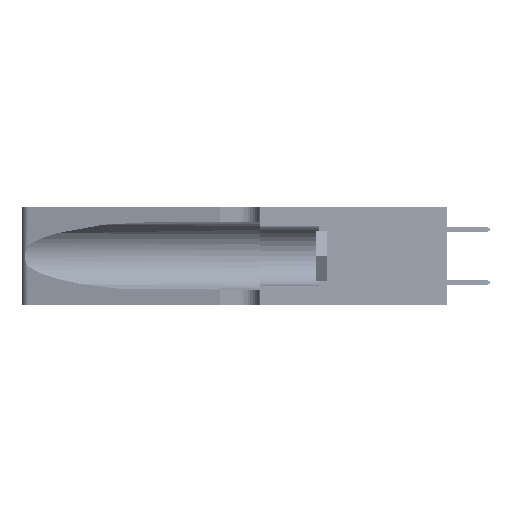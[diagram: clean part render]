
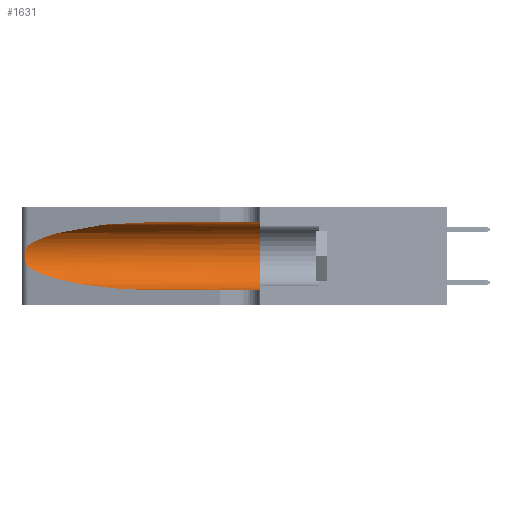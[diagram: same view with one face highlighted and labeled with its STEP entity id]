
A CAD part, left-side view. The second image highlights one B-rep face of the part: STEP entity #1631.
In plain terms, the highlighted cylindrical face has radius 3.308 mm (diameter 6.617 mm), a partial arc.
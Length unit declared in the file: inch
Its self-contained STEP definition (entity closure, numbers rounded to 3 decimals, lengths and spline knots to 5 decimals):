
#952 = CARTESIAN_POINT ( 'NONE',  ( 0.25487, 1.22718, 0.22369 ) ) ;
#1631 = ADVANCED_FACE ( 'NONE', ( #14194 ), #31816, .F. ) ;
#1812 = CARTESIAN_POINT ( 'NONE',  ( 0.1305, 0.72297, 0.31525 ) ) ;
#2856 = CARTESIAN_POINT ( 'NONE',  ( 0.2373, 1.15595, 0.08982 ) ) ;
#3126 = CIRCLE ( 'NONE', #28064, 0.13025 ) ;
#3781 = CARTESIAN_POINT ( 'NONE',  ( 0.25555, 1.22993, 0.14849 ) ) ;
#3948 = VECTOR ( 'NONE', #50388, 39.37008 ) ;
#4248 = ORIENTED_EDGE ( 'NONE', *, *, #35555, .F. ) ;
#6935 = CARTESIAN_POINT ( 'NONE',  ( 0.18966, 0.96281, 0.05475 ) ) ;
#7259 = LINE ( 'NONE', #22668, #47594 ) ;
#7669 = CARTESIAN_POINT ( 'NONE',  ( 0.25555, 1.22994, 0.2215 ) ) ;
#8319 = VERTEX_POINT ( 'NONE', #46606 ) ;
#9113 = DIRECTION ( 'NONE',  ( 0., -1., 0. ) ) ;
#9730 = DIRECTION ( 'NONE',  ( 0., 1., 0. ) ) ;
#11767 = CARTESIAN_POINT ( 'NONE',  ( 0.25787, 1.23484, 0.2124 ) ) ;
#12263 = CARTESIAN_POINT ( 'NONE',  ( 0.1305, 0.72297, 0.31525 ) ) ;
#12316 =( BOUNDED_CURVE ( )  B_SPLINE_CURVE ( 3, ( #12263, #40395, #44472, #20361 ),
 .UNSPECIFIED., .F., .F. ) 
 B_SPLINE_CURVE_WITH_KNOTS ( ( 4, 4 ),
 ( 1.5708, 2.84003 ),
 .UNSPECIFIED. ) 
 CURVE ( )  GEOMETRIC_REPRESENTATION_ITEM ( )  RATIONAL_B_SPLINE_CURVE ( ( 1., 0.87, 0.87, 1. ) ) 
 REPRESENTATION_ITEM ( '' )  );
#14194 = FACE_OUTER_BOUND ( 'NONE', #31170, .T. ) ;
#15791 = EDGE_CURVE ( 'NONE', #35054, #23074, #36114, .T. ) ;
#15822 = CARTESIAN_POINT ( 'NONE',  ( 0.26018, 1.23835, 0.19895 ) ) ;
#15950 = CARTESIAN_POINT ( 'NONE',  ( 0.1305, 0.35, 0.05475 ) ) ;
#16457 = VERTEX_POINT ( 'NONE', #1812 ) ;
#18172 = CARTESIAN_POINT ( 'NONE',  ( 0.1305, 1.61858, 0.05475 ) ) ;
#18825 = AXIS2_PLACEMENT_3D ( 'NONE', #25157, #9113, #37275 ) ;
#19876 = CARTESIAN_POINT ( 'NONE',  ( 0.26075, 1.23896, 0.178 ) ) ;
#20361 = CARTESIAN_POINT ( 'NONE',  ( 0.25487, 1.22718, 0.22369 ) ) ;
#22668 = CARTESIAN_POINT ( 'NONE',  ( 0.1305, 1.61858, 0.31525 ) ) ;
#23074 = VERTEX_POINT ( 'NONE', #15950 ) ;
#23900 = CARTESIAN_POINT ( 'NONE',  ( 0.25856, 1.23593, 0.16098 ) ) ;
#25157 = CARTESIAN_POINT ( 'NONE',  ( 0.1305, 1.61858, 0.185 ) ) ;
#25216 = EDGE_CURVE ( 'NONE', #48573, #51402, #40351, .T. ) ;
#26930 = ORIENTED_EDGE ( 'NONE', *, *, #41810, .T. ) ;
#27045 = CARTESIAN_POINT ( 'NONE',  ( 0.25487, 1.22718, 0.14631 ) ) ;
#27947 = CARTESIAN_POINT ( 'NONE',  ( 0.25639, 1.23186, 0.15144 ) ) ;
#28064 = AXIS2_PLACEMENT_3D ( 'NONE', #33852, #9730, #37884 ) ;
#28646 = EDGE_CURVE ( 'NONE', #16457, #48573, #12316, .T. ) ;
#30249 = EDGE_CURVE ( 'NONE', #16457, #8319, #7259, .T. ) ;
#30579 = DIRECTION ( 'NONE',  ( 0., -1., 0. ) ) ;
#31170 = EDGE_LOOP ( 'NONE', ( #37166, #31988, #26930, #39598, #4248, #35715 ) ) ;
#31816 = CYLINDRICAL_SURFACE ( 'NONE', #18825, 0.13025 ) ;
#31988 = ORIENTED_EDGE ( 'NONE', *, *, #25216, .T. ) ;
#32005 = CARTESIAN_POINT ( 'NONE',  ( 0.25487, 1.22718, 0.14631 ) ) ;
#33852 = CARTESIAN_POINT ( 'NONE',  ( 0.1305, 0.35, 0.185 ) ) ;
#35054 = VERTEX_POINT ( 'NONE', #46048 ) ;
#35140 = CARTESIAN_POINT ( 'NONE',  ( 0.1305, 0.72297, 0.05475 ) ) ;
#35555 = EDGE_CURVE ( 'NONE', #8319, #23074, #3126, .T. ) ;
#35715 = ORIENTED_EDGE ( 'NONE', *, *, #30249, .F. ) ;
#35857 = CARTESIAN_POINT ( 'NONE',  ( 0.25487, 1.22718, 0.22369 ) ) ;
#36114 = LINE ( 'NONE', #18172, #3948 ) ;
#37166 = ORIENTED_EDGE ( 'NONE', *, *, #28646, .T. ) ;
#37275 = DIRECTION ( 'NONE',  ( 0., 0., -1. ) ) ;
#37884 = DIRECTION ( 'NONE',  ( 0., 0., 1. ) ) ;
#39598 = ORIENTED_EDGE ( 'NONE', *, *, #15791, .T. ) ;
#39912 = CARTESIAN_POINT ( 'NONE',  ( 0.25854, 1.2359, 0.20912 ) ) ;
#40351 = B_SPLINE_CURVE_WITH_KNOTS ( 'NONE', 3,
 ( #35857, #7669, #47828, #11767, #39912, #15822, #43974, #19876, #48020, #23900, #52040, #27947, #3781, #32005 ),
 .UNSPECIFIED., .F., .F.,
 ( 4, 2, 2, 2, 2, 2, 4 ),
 ( 0., 0.00027, 0.00053, 0.00107, 0.0016, 0.00187, 0.00214 ),
 .UNSPECIFIED. ) ;
#40395 = CARTESIAN_POINT ( 'NONE',  ( 0.18966, 0.96281, 0.31525 ) ) ;
#41810 = EDGE_CURVE ( 'NONE', #51402, #35054, #45848, .T. ) ;
#43696 = CARTESIAN_POINT ( 'NONE',  ( 0.25487, 1.22718, 0.14631 ) ) ;
#43974 = CARTESIAN_POINT ( 'NONE',  ( 0.26075, 1.23896, 0.19203 ) ) ;
#44472 = CARTESIAN_POINT ( 'NONE',  ( 0.2373, 1.15595, 0.28018 ) ) ;
#45848 =( BOUNDED_CURVE ( )  B_SPLINE_CURVE ( 3, ( #27045, #2856, #6935, #35140 ),
 .UNSPECIFIED., .F., .T. ) 
 B_SPLINE_CURVE_WITH_KNOTS ( ( 4, 4 ),
 ( 3.44316, 4.71239 ),
 .UNSPECIFIED. ) 
 CURVE ( )  GEOMETRIC_REPRESENTATION_ITEM ( )  RATIONAL_B_SPLINE_CURVE ( ( 1., 0.87, 0.87, 1. ) ) 
 REPRESENTATION_ITEM ( '' )  );
#46048 = CARTESIAN_POINT ( 'NONE',  ( 0.1305, 0.72297, 0.05475 ) ) ;
#46606 = CARTESIAN_POINT ( 'NONE',  ( 0.1305, 0.35, 0.31525 ) ) ;
#47594 = VECTOR ( 'NONE', #30579, 39.37008 ) ;
#47828 = CARTESIAN_POINT ( 'NONE',  ( 0.25639, 1.23184, 0.21858 ) ) ;
#48020 = CARTESIAN_POINT ( 'NONE',  ( 0.26017, 1.23833, 0.17102 ) ) ;
#48573 = VERTEX_POINT ( 'NONE', #952 ) ;
#50388 = DIRECTION ( 'NONE',  ( 0., -1., 0. ) ) ;
#51402 = VERTEX_POINT ( 'NONE', #43696 ) ;
#52040 = CARTESIAN_POINT ( 'NONE',  ( 0.25789, 1.23486, 0.15765 ) ) ;
